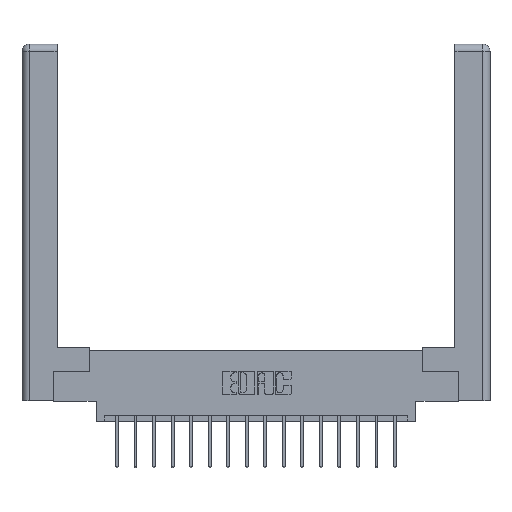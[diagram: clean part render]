
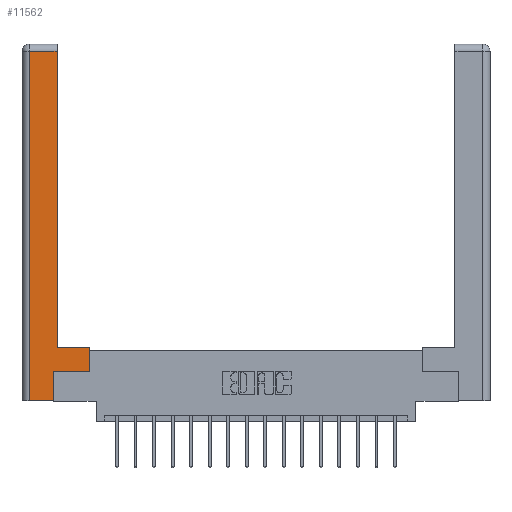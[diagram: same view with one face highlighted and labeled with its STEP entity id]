
A CAD part, top view. The second image highlights one B-rep face of the part: STEP entity #11562.
In plain terms, the highlighted planar face has unit normal (0, 0, 1).
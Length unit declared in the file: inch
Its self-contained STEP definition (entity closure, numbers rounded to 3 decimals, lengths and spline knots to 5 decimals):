
#667 = DIRECTION ( 'NONE',  ( -1., 0., 0. ) ) ;
#706 = ORIENTED_EDGE ( 'NONE', *, *, #9214, .T. ) ;
#1450 = FACE_OUTER_BOUND ( 'NONE', #8498, .T. ) ;
#1592 = ORIENTED_EDGE ( 'NONE', *, *, #17076, .T. ) ;
#1947 = CARTESIAN_POINT ( 'NONE',  ( 0., 0., 0. ) ) ;
#2286 = LINE ( 'NONE', #7300, #17056 ) ;
#2313 = CARTESIAN_POINT ( 'NONE',  ( 0.265, 0., 0. ) ) ;
#2706 = VECTOR ( 'NONE', #11579, 39.37008 ) ;
#2788 = VECTOR ( 'NONE', #4979, 39.37008 ) ;
#3066 = CARTESIAN_POINT ( 'NONE',  ( 0.265, 0., 0. ) ) ;
#3355 = VECTOR ( 'NONE', #12362, 39.37008 ) ;
#4202 = CARTESIAN_POINT ( 'NONE',  ( 0.565, 0.245, 0. ) ) ;
#4212 = LINE ( 'NONE', #15765, #17206 ) ;
#4390 = CARTESIAN_POINT ( 'NONE',  ( 0.265, 0.245, 0. ) ) ;
#4391 = LINE ( 'NONE', #15628, #14348 ) ;
#4978 = ORIENTED_EDGE ( 'NONE', *, *, #9779, .T. ) ;
#4979 = DIRECTION ( 'NONE',  ( -1., 0., 0. ) ) ;
#5037 = DIRECTION ( 'NONE',  ( 1., 0., 0. ) ) ;
#5124 = VERTEX_POINT ( 'NONE', #5649 ) ;
#5147 = VECTOR ( 'NONE', #15989, 39.37008 ) ;
#5379 = CARTESIAN_POINT ( 'NONE',  ( 0.565, 0.45, 0. ) ) ;
#5523 = DIRECTION ( 'NONE',  ( -1., 0., 0. ) ) ;
#5592 = LINE ( 'NONE', #10053, #5147 ) ;
#5645 = EDGE_CURVE ( 'NONE', #6065, #6623, #4212, .T. ) ;
#5649 = CARTESIAN_POINT ( 'NONE',  ( 0.0615, 0., 0. ) ) ;
#5771 = VECTOR ( 'NONE', #5037, 39.37008 ) ;
#5863 = AXIS2_PLACEMENT_3D ( 'NONE', #1947, #14981, #667 ) ;
#6065 = VERTEX_POINT ( 'NONE', #5379 ) ;
#6340 = VERTEX_POINT ( 'NONE', #3066 ) ;
#6623 = VERTEX_POINT ( 'NONE', #18028 ) ;
#7300 = CARTESIAN_POINT ( 'NONE',  ( 0.295, 3., 0. ) ) ;
#7361 = ORIENTED_EDGE ( 'NONE', *, *, #14572, .T. ) ;
#7970 = CARTESIAN_POINT ( 'NONE',  ( 0.0615, 2.94, 0. ) ) ;
#8498 = EDGE_LOOP ( 'NONE', ( #706, #1592, #10279, #9680, #4978, #7361, #9723, #18431 ) ) ;
#9034 = VERTEX_POINT ( 'NONE', #4202 ) ;
#9178 = EDGE_CURVE ( 'NONE', #9034, #6065, #13900, .T. ) ;
#9208 = VERTEX_POINT ( 'NONE', #17364 ) ;
#9214 = EDGE_CURVE ( 'NONE', #6623, #11058, #2286, .T. ) ;
#9531 = CARTESIAN_POINT ( 'NONE',  ( 0.295, 2.94, 0. ) ) ;
#9680 = ORIENTED_EDGE ( 'NONE', *, *, #15208, .T. ) ;
#9723 = ORIENTED_EDGE ( 'NONE', *, *, #9178, .T. ) ;
#9761 = DIRECTION ( 'NONE',  ( 0., -1., 0. ) ) ;
#9779 = EDGE_CURVE ( 'NONE', #6340, #12820, #5592, .T. ) ;
#10008 = DIRECTION ( 'NONE',  ( 0., 1., 0. ) ) ;
#10053 = CARTESIAN_POINT ( 'NONE',  ( 0.265, 0.245, 0. ) ) ;
#10133 = CARTESIAN_POINT ( 'NONE',  ( 0.565, 0.45, 0. ) ) ;
#10279 = ORIENTED_EDGE ( 'NONE', *, *, #11318, .T. ) ;
#10834 = LINE ( 'NONE', #7970, #2788 ) ;
#11058 = VERTEX_POINT ( 'NONE', #9531 ) ;
#11318 = EDGE_CURVE ( 'NONE', #9208, #5124, #4391, .T. ) ;
#11562 = ADVANCED_FACE ( 'NONE', ( #1450 ), #17666, .F. ) ;
#11579 = DIRECTION ( 'NONE',  ( 0., 1., 0. ) ) ;
#12362 = DIRECTION ( 'NONE',  ( 1., 0., 0. ) ) ;
#12546 = CARTESIAN_POINT ( 'NONE',  ( 0.565, 0.245, 0. ) ) ;
#12820 = VERTEX_POINT ( 'NONE', #4390 ) ;
#13625 = LINE ( 'NONE', #2313, #5771 ) ;
#13900 = LINE ( 'NONE', #10133, #2706 ) ;
#14348 = VECTOR ( 'NONE', #9761, 39.37008 ) ;
#14572 = EDGE_CURVE ( 'NONE', #12820, #9034, #16581, .T. ) ;
#14981 = DIRECTION ( 'NONE',  ( 0., 0., -1. ) ) ;
#15208 = EDGE_CURVE ( 'NONE', #5124, #6340, #13625, .T. ) ;
#15628 = CARTESIAN_POINT ( 'NONE',  ( 0.0615, 0., 0. ) ) ;
#15765 = CARTESIAN_POINT ( 'NONE',  ( 0.295, 0.45, 0. ) ) ;
#15989 = DIRECTION ( 'NONE',  ( 0., 1., 0. ) ) ;
#16581 = LINE ( 'NONE', #12546, #3355 ) ;
#17056 = VECTOR ( 'NONE', #10008, 39.37008 ) ;
#17076 = EDGE_CURVE ( 'NONE', #11058, #9208, #10834, .T. ) ;
#17206 = VECTOR ( 'NONE', #5523, 39.37008 ) ;
#17364 = CARTESIAN_POINT ( 'NONE',  ( 0.0615, 2.94, 0. ) ) ;
#17666 = PLANE ( 'NONE',  #5863 ) ;
#18028 = CARTESIAN_POINT ( 'NONE',  ( 0.295, 0.45, 0. ) ) ;
#18431 = ORIENTED_EDGE ( 'NONE', *, *, #5645, .T. ) ;
